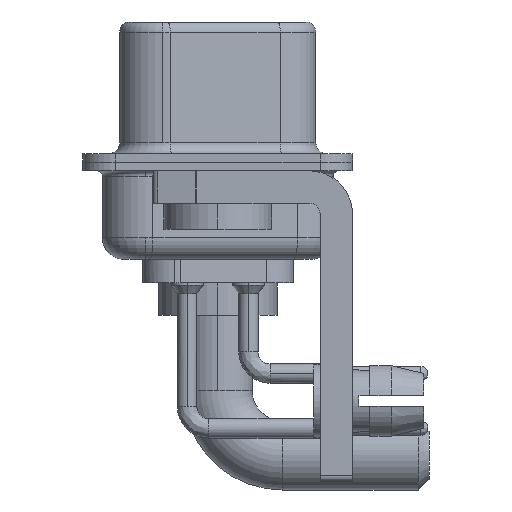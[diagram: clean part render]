
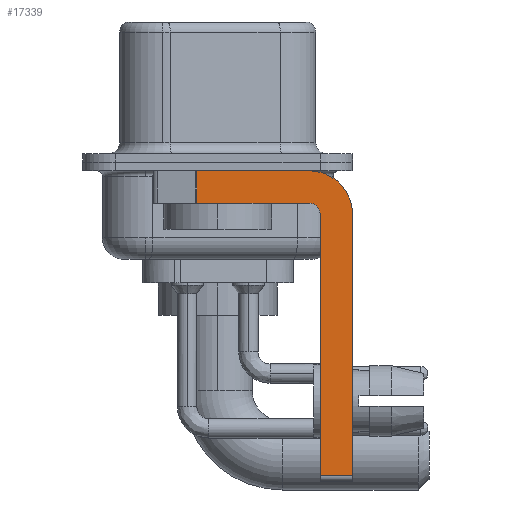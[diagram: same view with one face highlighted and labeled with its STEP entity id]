
A CAD part, left-side view. The second image highlights one B-rep face of the part: STEP entity #17339.
In plain terms, the highlighted planar face has unit normal (-1, 0, 0).
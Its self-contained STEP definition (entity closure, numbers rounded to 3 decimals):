
#106 = EDGE_CURVE ( 'NONE', #12977, #21393, #11205, .T. ) ;
#258 = CARTESIAN_POINT ( 'NONE',  ( -2.9, -4.25, -1.9 ) ) ;
#826 = ORIENTED_EDGE ( 'NONE', *, *, #879, .T. ) ;
#871 = VECTOR ( 'NONE', #19935, 1000. ) ;
#879 = EDGE_CURVE ( 'NONE', #16236, #15239, #17338, .T. ) ;
#1001 = PLANE ( 'NONE',  #16934 ) ;
#1728 = ORIENTED_EDGE ( 'NONE', *, *, #13215, .F. ) ;
#2052 = CIRCLE ( 'NONE', #12181, 0.5 ) ;
#2200 = EDGE_CURVE ( 'NONE', #5174, #15239, #25819, .T. ) ;
#2367 = LINE ( 'NONE', #11164, #871 ) ;
#2700 = AXIS2_PLACEMENT_3D ( 'NONE', #15963, #13662, #22433 ) ;
#3302 = DIRECTION ( 'NONE',  ( 0., 0., -1. ) ) ;
#4663 = ORIENTED_EDGE ( 'NONE', *, *, #23553, .F. ) ;
#4805 = LINE ( 'NONE', #6848, #13871 ) ;
#5173 = DIRECTION ( 'NONE',  ( 1., 0., 0. ) ) ;
#5174 = VERTEX_POINT ( 'NONE', #21478 ) ;
#5258 = VECTOR ( 'NONE', #6383, 1000. ) ;
#5951 = CARTESIAN_POINT ( 'NONE',  ( -2.9, -6.25, -2.4 ) ) ;
#6383 = DIRECTION ( 'NONE',  ( 0., -1., 0. ) ) ;
#6386 = DIRECTION ( 'NONE',  ( 0., 0., 1. ) ) ;
#6665 = DIRECTION ( 'NONE',  ( -1., 0., 0. ) ) ;
#6848 = CARTESIAN_POINT ( 'NONE',  ( -2.9, 3., -0.4 ) ) ;
#7381 = VERTEX_POINT ( 'NONE', #20859 ) ;
#9631 = ORIENTED_EDGE ( 'NONE', *, *, #18076, .F. ) ;
#9905 = VECTOR ( 'NONE', #23641, 1000. ) ;
#11054 = CARTESIAN_POINT ( 'NONE',  ( -2.9, -4.75, -14.55 ) ) ;
#11164 = CARTESIAN_POINT ( 'NONE',  ( -2.9, -4.75, -14.8 ) ) ;
#11205 = LINE ( 'NONE', #258, #13725 ) ;
#11630 = EDGE_LOOP ( 'NONE', ( #17436, #23653, #22371, #1728, #9631, #826, #19728, #4663 ) ) ;
#12155 = CARTESIAN_POINT ( 'NONE',  ( -2.9, -6.25, -14.55 ) ) ;
#12181 = AXIS2_PLACEMENT_3D ( 'NONE', #19482, #6665, #6386 ) ;
#12977 = VERTEX_POINT ( 'NONE', #24838 ) ;
#13215 = EDGE_CURVE ( 'NONE', #22826, #12977, #2052, .T. ) ;
#13614 = DIRECTION ( 'NONE',  ( 0., -1., 0. ) ) ;
#13662 = DIRECTION ( 'NONE',  ( 1., 0., 0. ) ) ;
#13725 = VECTOR ( 'NONE', #22431, 1000. ) ;
#13868 = CARTESIAN_POINT ( 'NONE',  ( -2.9, -4.75, -2.4 ) ) ;
#13871 = VECTOR ( 'NONE', #13614, 1000. ) ;
#15239 = VERTEX_POINT ( 'NONE', #12155 ) ;
#15415 = DIRECTION ( 'NONE',  ( 0., 0., -1. ) ) ;
#15963 = CARTESIAN_POINT ( 'NONE',  ( -2.9, -4.25, -2.4 ) ) ;
#16236 = VERTEX_POINT ( 'NONE', #11054 ) ;
#16252 = VERTEX_POINT ( 'NONE', #22124 ) ;
#16934 = AXIS2_PLACEMENT_3D ( 'NONE', #24905, #5173, #3302 ) ;
#17338 = LINE ( 'NONE', #26109, #5258 ) ;
#17339 = ADVANCED_FACE ( 'NONE', ( #25326 ), #1001, .F. ) ;
#17436 = ORIENTED_EDGE ( 'NONE', *, *, #20735, .F. ) ;
#17448 = LINE ( 'NONE', #18014, #24682 ) ;
#18014 = CARTESIAN_POINT ( 'NONE',  ( -2.9, 0.978, -1.9 ) ) ;
#18076 = EDGE_CURVE ( 'NONE', #16236, #22826, #2367, .T. ) ;
#18329 = CARTESIAN_POINT ( 'NONE',  ( -2.9, 0.978, -1.9 ) ) ;
#19482 = CARTESIAN_POINT ( 'NONE',  ( -2.9, -4.25, -2.4 ) ) ;
#19728 = ORIENTED_EDGE ( 'NONE', *, *, #2200, .F. ) ;
#19935 = DIRECTION ( 'NONE',  ( 0., 0., 1. ) ) ;
#20735 = EDGE_CURVE ( 'NONE', #7381, #16252, #4805, .T. ) ;
#20859 = CARTESIAN_POINT ( 'NONE',  ( -2.9, 0.978, -0.4 ) ) ;
#21393 = VERTEX_POINT ( 'NONE', #18329 ) ;
#21478 = CARTESIAN_POINT ( 'NONE',  ( -2.9, -6.25, -2.4 ) ) ;
#21674 = EDGE_CURVE ( 'NONE', #7381, #21393, #17448, .T. ) ;
#22124 = CARTESIAN_POINT ( 'NONE',  ( -2.9, -4.25, -0.4 ) ) ;
#22371 = ORIENTED_EDGE ( 'NONE', *, *, #106, .F. ) ;
#22431 = DIRECTION ( 'NONE',  ( 0., 1., 0. ) ) ;
#22433 = DIRECTION ( 'NONE',  ( 0., 0., -1. ) ) ;
#22826 = VERTEX_POINT ( 'NONE', #13868 ) ;
#23553 = EDGE_CURVE ( 'NONE', #16252, #5174, #23844, .T. ) ;
#23641 = DIRECTION ( 'NONE',  ( 0., 0., -1. ) ) ;
#23653 = ORIENTED_EDGE ( 'NONE', *, *, #21674, .T. ) ;
#23844 = CIRCLE ( 'NONE', #2700, 2. ) ;
#24682 = VECTOR ( 'NONE', #15415, 1000. ) ;
#24838 = CARTESIAN_POINT ( 'NONE',  ( -2.9, -4.25, -1.9 ) ) ;
#24905 = CARTESIAN_POINT ( 'NONE',  ( -2.9, -4.25, -2.4 ) ) ;
#25326 = FACE_OUTER_BOUND ( 'NONE', #11630, .T. ) ;
#25819 = LINE ( 'NONE', #5951, #9905 ) ;
#26109 = CARTESIAN_POINT ( 'NONE',  ( -2.9, -4.25, -14.55 ) ) ;
